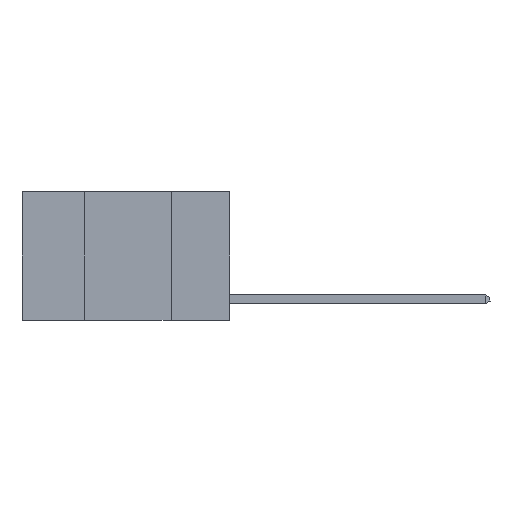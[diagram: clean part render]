
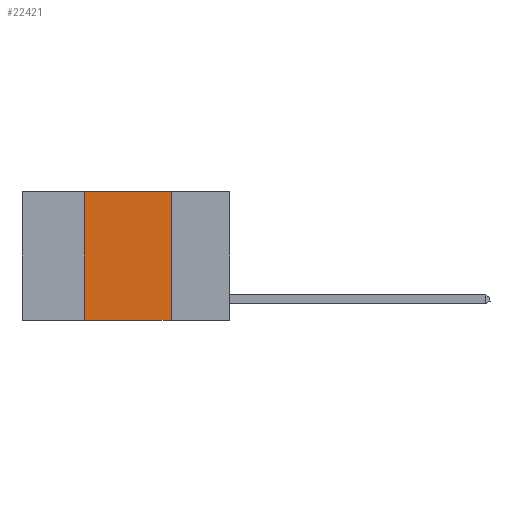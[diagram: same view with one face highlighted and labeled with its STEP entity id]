
A CAD part, left-side view. The second image highlights one B-rep face of the part: STEP entity #22421.
In plain terms, the highlighted planar face has unit normal (-1, 0, 0).
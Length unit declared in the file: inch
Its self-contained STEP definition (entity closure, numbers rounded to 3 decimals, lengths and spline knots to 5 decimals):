
#250 = ORIENTED_EDGE ( 'NONE', *, *, #16210, .F. ) ;
#937 = ORIENTED_EDGE ( 'NONE', *, *, #25911, .T. ) ;
#948 = CARTESIAN_POINT ( 'NONE',  ( 0., 0.17, 0. ) ) ;
#1581 = LINE ( 'NONE', #20482, #5176 ) ;
#2106 = LINE ( 'NONE', #25023, #7615 ) ;
#2412 = VERTEX_POINT ( 'NONE', #17986 ) ;
#3189 = VERTEX_POINT ( 'NONE', #8074 ) ;
#4704 = FACE_OUTER_BOUND ( 'NONE', #25854, .T. ) ;
#5176 = VECTOR ( 'NONE', #22553, 39.37008 ) ;
#5588 = PLANE ( 'NONE',  #26298 ) ;
#7615 = VECTOR ( 'NONE', #12786, 39.37008 ) ;
#7630 = DIRECTION ( 'NONE',  ( 0., 0., -1. ) ) ;
#8074 = CARTESIAN_POINT ( 'NONE',  ( 0., 0.17, -0.37 ) ) ;
#9396 = ORIENTED_EDGE ( 'NONE', *, *, #19667, .F. ) ;
#11333 = VECTOR ( 'NONE', #16118, 39.37008 ) ;
#11397 = DIRECTION ( 'NONE',  ( 0., 0., -1. ) ) ;
#12786 = DIRECTION ( 'NONE',  ( 0., -1., 0. ) ) ;
#12890 = VERTEX_POINT ( 'NONE', #16751 ) ;
#16118 = DIRECTION ( 'NONE',  ( 0., -1., 0. ) ) ;
#16210 = EDGE_CURVE ( 'NONE', #17214, #12890, #1581, .T. ) ;
#16751 = CARTESIAN_POINT ( 'NONE',  ( 0., 0.42, 0. ) ) ;
#17214 = VERTEX_POINT ( 'NONE', #25709 ) ;
#17688 = VECTOR ( 'NONE', #11397, 39.37008 ) ;
#17863 = CARTESIAN_POINT ( 'NONE',  ( 0., 0.6, 0. ) ) ;
#17986 = CARTESIAN_POINT ( 'NONE',  ( 0., 0.17, 0. ) ) ;
#18241 = EDGE_CURVE ( 'NONE', #12890, #2412, #2106, .T. ) ;
#19667 = EDGE_CURVE ( 'NONE', #2412, #3189, #23139, .T. ) ;
#19934 = DIRECTION ( 'NONE',  ( 1., 0., 0. ) ) ;
#20482 = CARTESIAN_POINT ( 'NONE',  ( 0., 0.42, 0. ) ) ;
#21573 = LINE ( 'NONE', #26315, #11333 ) ;
#21583 = ORIENTED_EDGE ( 'NONE', *, *, #18241, .F. ) ;
#22421 = ADVANCED_FACE ( 'NONE', ( #4704 ), #5588, .F. ) ;
#22553 = DIRECTION ( 'NONE',  ( 0., 0., 1. ) ) ;
#23139 = LINE ( 'NONE', #948, #17688 ) ;
#25023 = CARTESIAN_POINT ( 'NONE',  ( 0., 0.6, 0. ) ) ;
#25709 = CARTESIAN_POINT ( 'NONE',  ( 0., 0.42, -0.37 ) ) ;
#25854 = EDGE_LOOP ( 'NONE', ( #9396, #21583, #250, #937 ) ) ;
#25911 = EDGE_CURVE ( 'NONE', #17214, #3189, #21573, .T. ) ;
#26298 = AXIS2_PLACEMENT_3D ( 'NONE', #17863, #19934, #7630 ) ;
#26315 = CARTESIAN_POINT ( 'NONE',  ( 0., 0.6, -0.37 ) ) ;
